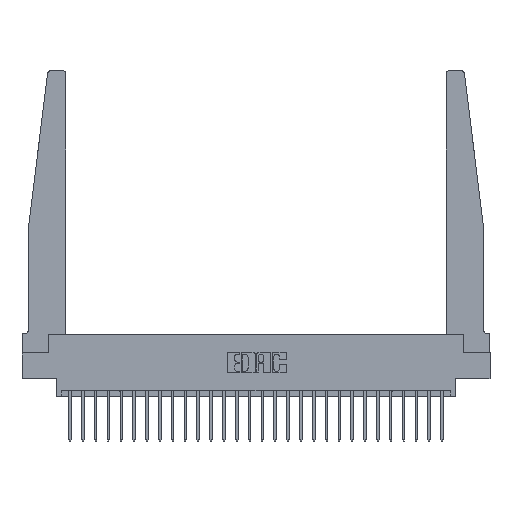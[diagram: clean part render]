
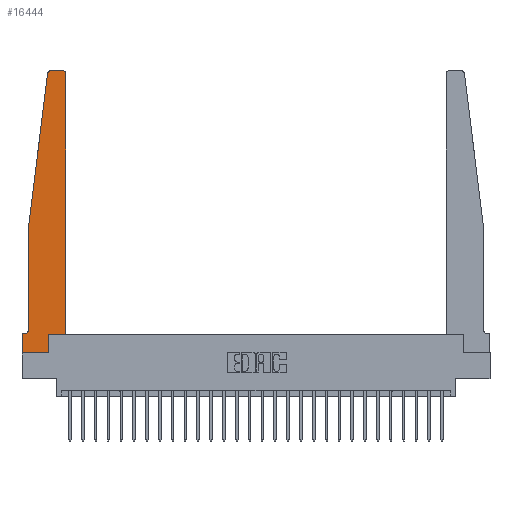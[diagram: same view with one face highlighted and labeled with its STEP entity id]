
A CAD part, top view. The second image highlights one B-rep face of the part: STEP entity #16444.
In plain terms, the highlighted planar face has unit normal (0, 0, 1).
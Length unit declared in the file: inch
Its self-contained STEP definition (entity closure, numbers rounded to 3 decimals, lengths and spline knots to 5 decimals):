
#122 = DIRECTION ( 'NONE',  ( -1., 0., 0. ) ) ;
#355 = ORIENTED_EDGE ( 'NONE', *, *, #19845, .T. ) ;
#961 = PLANE ( 'NONE',  #19373 ) ;
#976 = ORIENTED_EDGE ( 'NONE', *, *, #12570, .T. ) ;
#1373 = DIRECTION ( 'NONE',  ( -0.122, -0.992, 0. ) ) ;
#1552 = LINE ( 'NONE', #8105, #4896 ) ;
#1644 = CARTESIAN_POINT ( 'NONE',  ( 0., 0., 0.37 ) ) ;
#1892 = CARTESIAN_POINT ( 'NONE',  ( 0.065, 1.25, 0.37 ) ) ;
#2096 = VECTOR ( 'NONE', #10724, 39.37008 ) ;
#2255 = CARTESIAN_POINT ( 'NONE',  ( 0.425, 0.18, 0.37 ) ) ;
#2312 = EDGE_CURVE ( 'NONE', #8645, #23898, #1552, .T. ) ;
#2590 = ORIENTED_EDGE ( 'NONE', *, *, #22324, .T. ) ;
#3037 = VERTEX_POINT ( 'NONE', #19367 ) ;
#3429 = DIRECTION ( 'NONE',  ( 0., 1., 0. ) ) ;
#3434 = CARTESIAN_POINT ( 'NONE',  ( 0.425, 0.18, 0.37 ) ) ;
#3630 = DIRECTION ( 'NONE',  ( -1., 0., 0. ) ) ;
#3859 = LINE ( 'NONE', #22537, #11924 ) ;
#3903 = LINE ( 'NONE', #1892, #23140 ) ;
#4003 = DIRECTION ( 'NONE',  ( -1., 0., 0. ) ) ;
#4551 = CARTESIAN_POINT ( 'NONE',  ( 0.065, 1.25, 0.37 ) ) ;
#4702 = CARTESIAN_POINT ( 'NONE',  ( 0.24675, 2.72367, 0.37 ) ) ;
#4896 = VECTOR ( 'NONE', #3429, 39.37008 ) ;
#4903 = VERTEX_POINT ( 'NONE', #15066 ) ;
#5249 = DIRECTION ( 'NONE',  ( 1., 0., 0. ) ) ;
#5777 = ORIENTED_EDGE ( 'NONE', *, *, #18418, .T. ) ;
#5789 = VECTOR ( 'NONE', #9832, 39.37008 ) ;
#6285 = VERTEX_POINT ( 'NONE', #4702 ) ;
#6475 = EDGE_LOOP ( 'NONE', ( #13371, #16931, #2590, #8185, #18695, #976, #10734, #20937, #355, #5777, #24754, #16900 ) ) ;
#6813 = VERTEX_POINT ( 'NONE', #23682 ) ;
#7665 = CARTESIAN_POINT ( 'NONE',  ( 0.27653, 2.72, 0.37 ) ) ;
#7968 = EDGE_CURVE ( 'NONE', #10547, #17429, #21237, .T. ) ;
#8105 = CARTESIAN_POINT ( 'NONE',  ( 0.425, 0.18, 0.37 ) ) ;
#8185 = ORIENTED_EDGE ( 'NONE', *, *, #7968, .T. ) ;
#8547 = LINE ( 'NONE', #12712, #11471 ) ;
#8645 = VERTEX_POINT ( 'NONE', #3434 ) ;
#9218 = CARTESIAN_POINT ( 'NONE',  ( 0.015, 0.1875, 0.37 ) ) ;
#9832 = DIRECTION ( 'NONE',  ( 1., 0., 0. ) ) ;
#10547 = VERTEX_POINT ( 'NONE', #23276 ) ;
#10724 = DIRECTION ( 'NONE',  ( 0., -1., 0. ) ) ;
#10734 = ORIENTED_EDGE ( 'NONE', *, *, #24843, .T. ) ;
#10855 = CARTESIAN_POINT ( 'NONE',  ( 0.015, 0.2375, 0.37 ) ) ;
#11227 = VERTEX_POINT ( 'NONE', #20779 ) ;
#11465 = CIRCLE ( 'NONE', #26507, 0.03 ) ;
#11471 = VECTOR ( 'NONE', #4003, 39.37008 ) ;
#11924 = VECTOR ( 'NONE', #18193, 39.37008 ) ;
#12371 = AXIS2_PLACEMENT_3D ( 'NONE', #14085, #26326, #16099 ) ;
#12570 = EDGE_CURVE ( 'NONE', #24096, #25917, #8547, .T. ) ;
#12712 = CARTESIAN_POINT ( 'NONE',  ( 0.065, 0.1875, 0.37 ) ) ;
#13176 = VECTOR ( 'NONE', #19025, 39.37008 ) ;
#13274 = EDGE_CURVE ( 'NONE', #4903, #23549, #24455, .T. ) ;
#13313 = DIRECTION ( 'NONE',  ( 0., 0., 1. ) ) ;
#13371 = ORIENTED_EDGE ( 'NONE', *, *, #13274, .T. ) ;
#13848 = DIRECTION ( 'NONE',  ( 0., 0., 1. ) ) ;
#14085 = CARTESIAN_POINT ( 'NONE',  ( 0.395, 2.72, 0.37 ) ) ;
#14147 = CARTESIAN_POINT ( 'NONE',  ( 0., 0., 0.37 ) ) ;
#14343 = CARTESIAN_POINT ( 'NONE',  ( 0.425, 2.72, 0.37 ) ) ;
#15066 = CARTESIAN_POINT ( 'NONE',  ( 0.395, 2.75, 0.37 ) ) ;
#15398 = EDGE_CURVE ( 'NONE', #17429, #24096, #25436, .T. ) ;
#15845 = CARTESIAN_POINT ( 'NONE',  ( 0.25, 2.75, 0.37 ) ) ;
#16099 = DIRECTION ( 'NONE',  ( 1., 0., 0. ) ) ;
#16213 = LINE ( 'NONE', #2255, #13176 ) ;
#16444 = ADVANCED_FACE ( 'NONE', ( #21654 ), #961, .T. ) ;
#16900 = ORIENTED_EDGE ( 'NONE', *, *, #19656, .T. ) ;
#16931 = ORIENTED_EDGE ( 'NONE', *, *, #20815, .T. ) ;
#17017 = DIRECTION ( 'NONE',  ( 0., 0., -1. ) ) ;
#17429 = VERTEX_POINT ( 'NONE', #22127 ) ;
#18193 = DIRECTION ( 'NONE',  ( 0., 1., 0. ) ) ;
#18418 = EDGE_CURVE ( 'NONE', #3037, #8645, #16213, .T. ) ;
#18695 = ORIENTED_EDGE ( 'NONE', *, *, #15398, .T. ) ;
#19025 = DIRECTION ( 'NONE',  ( 1., 0., 0. ) ) ;
#19367 = CARTESIAN_POINT ( 'NONE',  ( 0.2605, 0.18, 0.37 ) ) ;
#19373 = AXIS2_PLACEMENT_3D ( 'NONE', #26077, #13313, #5249 ) ;
#19656 = EDGE_CURVE ( 'NONE', #23898, #4903, #24840, .T. ) ;
#19845 = EDGE_CURVE ( 'NONE', #6813, #3037, #3859, .T. ) ;
#20037 = LINE ( 'NONE', #1644, #5789 ) ;
#20067 = LINE ( 'NONE', #14147, #20835 ) ;
#20312 = DIRECTION ( 'NONE',  ( 1., 0., 0. ) ) ;
#20779 = CARTESIAN_POINT ( 'NONE',  ( 0., 0., 0.37 ) ) ;
#20815 = EDGE_CURVE ( 'NONE', #23549, #6285, #11465, .T. ) ;
#20835 = VECTOR ( 'NONE', #22372, 39.37008 ) ;
#20937 = ORIENTED_EDGE ( 'NONE', *, *, #25328, .T. ) ;
#21237 = LINE ( 'NONE', #4551, #2096 ) ;
#21654 = FACE_OUTER_BOUND ( 'NONE', #6475, .T. ) ;
#22127 = CARTESIAN_POINT ( 'NONE',  ( 0.065, 0.2375, 0.37 ) ) ;
#22324 = EDGE_CURVE ( 'NONE', #6285, #10547, #3903, .T. ) ;
#22372 = DIRECTION ( 'NONE',  ( 0., -1., 0. ) ) ;
#22537 = CARTESIAN_POINT ( 'NONE',  ( 0.2605, 0.18, 0.37 ) ) ;
#22656 = VECTOR ( 'NONE', #3630, 39.37008 ) ;
#23140 = VECTOR ( 'NONE', #1373, 39.37008 ) ;
#23276 = CARTESIAN_POINT ( 'NONE',  ( 0.065, 1.25, 0.37 ) ) ;
#23549 = VERTEX_POINT ( 'NONE', #25009 ) ;
#23682 = CARTESIAN_POINT ( 'NONE',  ( 0.2605, 0., 0.37 ) ) ;
#23898 = VERTEX_POINT ( 'NONE', #14343 ) ;
#24096 = VERTEX_POINT ( 'NONE', #9218 ) ;
#24455 = LINE ( 'NONE', #15845, #22656 ) ;
#24754 = ORIENTED_EDGE ( 'NONE', *, *, #2312, .T. ) ;
#24840 = CIRCLE ( 'NONE', #12371, 0.03 ) ;
#24843 = EDGE_CURVE ( 'NONE', #25917, #11227, #20067, .T. ) ;
#25006 = AXIS2_PLACEMENT_3D ( 'NONE', #10855, #17017, #122 ) ;
#25009 = CARTESIAN_POINT ( 'NONE',  ( 0.27653, 2.75, 0.37 ) ) ;
#25328 = EDGE_CURVE ( 'NONE', #11227, #6813, #20037, .T. ) ;
#25436 = CIRCLE ( 'NONE', #25006, 0.05 ) ;
#25481 = CARTESIAN_POINT ( 'NONE',  ( 0., 0.1875, 0.37 ) ) ;
#25917 = VERTEX_POINT ( 'NONE', #25481 ) ;
#26077 = CARTESIAN_POINT ( 'NONE',  ( 0., 0.1875, 0.37 ) ) ;
#26326 = DIRECTION ( 'NONE',  ( 0., 0., 1. ) ) ;
#26507 = AXIS2_PLACEMENT_3D ( 'NONE', #7665, #13848, #20312 ) ;
